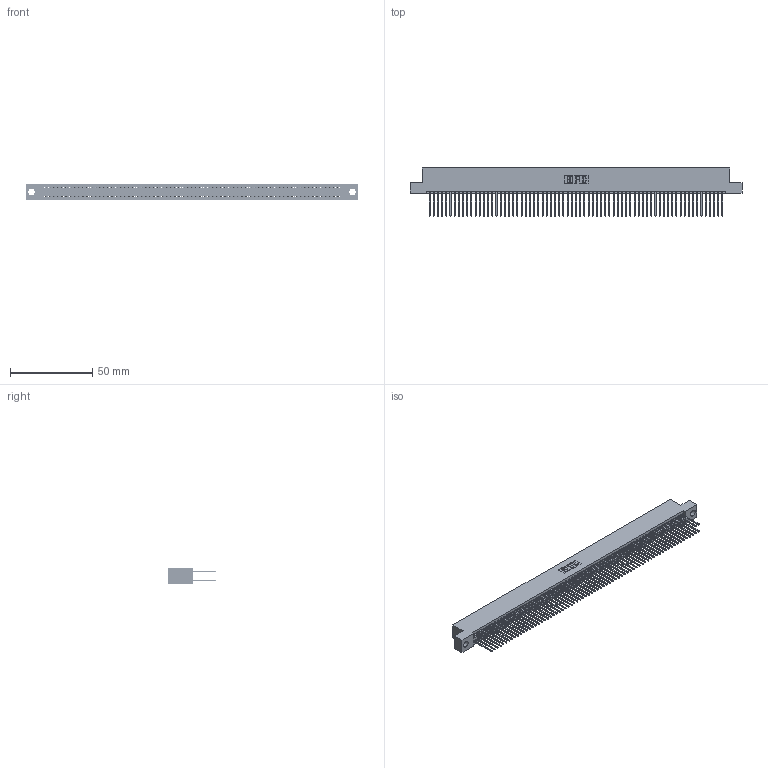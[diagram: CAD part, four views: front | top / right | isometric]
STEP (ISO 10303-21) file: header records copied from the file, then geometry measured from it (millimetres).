
FILE_DESCRIPTION (( 'STEP AP203' ), '1' );
FILE_NAME ('395-142-540-204.STEP', '2021-06-18T05:18:51', ( '' ), ( '' ), 'SwSTEP 2.0', 'SolidWorks 2020', '' );
FILE_SCHEMA (( 'CONFIG_CONTROL_DESIGN' ));
Length unit declared in the file: inch
Products named in the file (3): 345-292-001_345-293-140; 395-142-540-204; 345 Part_Flush Mounting Lugs - 0.156 Dia-TI
Assembly tree (143 placements, depth 2):
  395-142-540-204
    345 Part_Flush Mounting Lugs - 0.156 Dia-TI
    345-292-001_345-293-140  x142
Bounding box: 201.55 x 29.13 x 9.4 mm (x, y, z)
Volume: 20280.2 mm3; surface area: 32888.3 mm2
Topology: 143 solids, 143 shells, 7240 faces, 21535 edges, 14166 vertices
Faces by surface type: plane 4780, cylinder 2460
Entity records: 52241 total; most frequent: CARTESIAN_POINT 8734, ORIENTED_EDGE 8666, DIRECTION 7665, EDGE_CURVE 4333, VECTOR 3917, LINE 3917, VERTEX_POINT 2886, AXIS2_PLACEMENT_3D 1874
